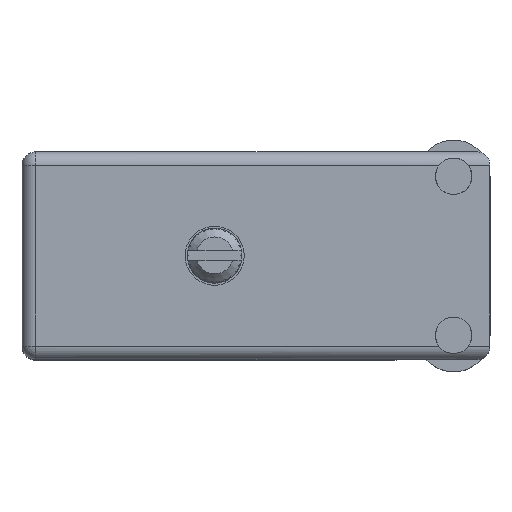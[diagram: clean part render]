
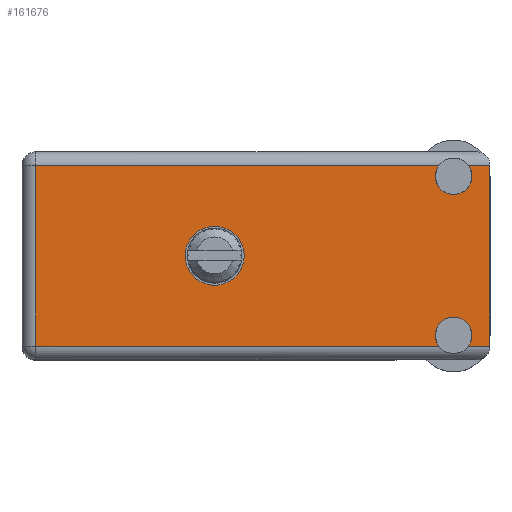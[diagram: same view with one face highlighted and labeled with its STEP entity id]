
A CAD part, top view. The second image highlights one B-rep face of the part: STEP entity #161676.
In plain terms, the highlighted face is planar.
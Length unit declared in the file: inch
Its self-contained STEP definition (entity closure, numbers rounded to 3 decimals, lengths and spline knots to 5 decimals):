
#1662 = DIRECTION ( 'NONE',  ( 1., 0., 0. ) ) ;
#2091 = VECTOR ( 'NONE', #37955, 39.37008 ) ;
#2223 = CIRCLE ( 'NONE', #14769, 0.1015 ) ;
#3680 = DIRECTION ( 'NONE',  ( 0., 0., 1. ) ) ;
#5959 = VERTEX_POINT ( 'NONE', #51425 ) ;
#6111 = FACE_BOUND ( 'NONE', #151323, .T. ) ;
#6611 = CARTESIAN_POINT ( 'NONE',  ( 1.484, 0.906, -0.084 ) ) ;
#6957 = CARTESIAN_POINT ( 'NONE',  ( 1.53437, 0.906, -0.668 ) ) ;
#7095 = DIRECTION ( 'NONE',  ( -1., 0., 0. ) ) ;
#10945 = EDGE_CURVE ( 'NONE', #169000, #53240, #169586, .T. ) ;
#13604 = ORIENTED_EDGE ( 'NONE', *, *, #43337, .T. ) ;
#13676 = CARTESIAN_POINT ( 'NONE',  ( 1.484, 0.906, -0.1465 ) ) ;
#14152 = EDGE_CURVE ( 'NONE', #182163, #169000, #41127, .T. ) ;
#14405 = AXIS2_PLACEMENT_3D ( 'NONE', #101780, #162920, #118537 ) ;
#14769 = AXIS2_PLACEMENT_3D ( 'NONE', #75644, #45050, #132971 ) ;
#16788 = CIRCLE ( 'NONE', #189919, 0.0625 ) ;
#18966 = DIRECTION ( 'NONE',  ( 0., 0., 1. ) ) ;
#21235 = DIRECTION ( 'NONE',  ( 0., 0., 1. ) ) ;
#26805 = AXIS2_PLACEMENT_3D ( 'NONE', #66387, #154219, #18966 ) ;
#27345 = DIRECTION ( 'NONE',  ( 1., 0., 0. ) ) ;
#29380 = CARTESIAN_POINT ( 'NONE',  ( 1.609, 0.906, -0.047 ) ) ;
#34999 = CARTESIAN_POINT ( 'NONE',  ( 0.047, 0.906, -0.715 ) ) ;
#36084 = DIRECTION ( 'NONE',  ( 0., 1., 0. ) ) ;
#37955 = DIRECTION ( 'NONE',  ( 0., 0., 1. ) ) ;
#38974 = CARTESIAN_POINT ( 'NONE',  ( 0.047, 0.906, -0.668 ) ) ;
#39924 = CIRCLE ( 'NONE', #125039, 0.1015 ) ;
#40040 = ORIENTED_EDGE ( 'NONE', *, *, #151845, .F. ) ;
#41127 = CIRCLE ( 'NONE', #79023, 0.0625 ) ;
#43337 = EDGE_CURVE ( 'NONE', #182163, #186503, #110846, .T. ) ;
#44783 = DIRECTION ( 'NONE',  ( 0., 1., 0. ) ) ;
#45050 = DIRECTION ( 'NONE',  ( 0., 1., 0. ) ) ;
#45197 = EDGE_CURVE ( 'NONE', #61431, #184774, #151283, .T. ) ;
#45761 = DIRECTION ( 'NONE',  ( 0., 0., 1. ) ) ;
#49197 = VERTEX_POINT ( 'NONE', #66210 ) ;
#49607 = FACE_OUTER_BOUND ( 'NONE', #87204, .T. ) ;
#50571 = CARTESIAN_POINT ( 'NONE',  ( 0.6625, 0.906, -0.256 ) ) ;
#51425 = CARTESIAN_POINT ( 'NONE',  ( 1.609, 0.906, -0.047 ) ) ;
#51627 = DIRECTION ( 'NONE',  ( 0., 1., 0. ) ) ;
#51760 = LINE ( 'NONE', #34999, #2091 ) ;
#53240 = VERTEX_POINT ( 'NONE', #6957 ) ;
#54819 = DIRECTION ( 'NONE',  ( -1., 0., 0. ) ) ;
#59833 = VECTOR ( 'NONE', #7095, 39.37008 ) ;
#61431 = VERTEX_POINT ( 'NONE', #144562 ) ;
#61825 = VERTEX_POINT ( 'NONE', #50571 ) ;
#61921 = EDGE_CURVE ( 'NONE', #184774, #67930, #16788, .T. ) ;
#63448 = ORIENTED_EDGE ( 'NONE', *, *, #10945, .F. ) ;
#66210 = CARTESIAN_POINT ( 'NONE',  ( 0.047, 0.906, -0.047 ) ) ;
#66387 = CARTESIAN_POINT ( 'NONE',  ( 0., 0.906, -0.715 ) ) ;
#67930 = VERTEX_POINT ( 'NONE', #141835 ) ;
#70359 = CARTESIAN_POINT ( 'NONE',  ( 1.484, 0.906, -0.084 ) ) ;
#73168 = ORIENTED_EDGE ( 'NONE', *, *, #86014, .F. ) ;
#75644 = CARTESIAN_POINT ( 'NONE',  ( 0.6625, 0.906, -0.3575 ) ) ;
#76755 = LINE ( 'NONE', #29380, #187191 ) ;
#79023 = AXIS2_PLACEMENT_3D ( 'NONE', #184131, #36084, #21235 ) ;
#84676 = CARTESIAN_POINT ( 'NONE',  ( 1.609, 0.906, -0.047 ) ) ;
#86014 = EDGE_CURVE ( 'NONE', #150300, #5959, #179741, .T. ) ;
#87204 = EDGE_LOOP ( 'NONE', ( #182590, #155011, #193056, #114177, #73168, #184280, #63448, #105481, #13604, #168948 ) ) ;
#88537 = EDGE_CURVE ( 'NONE', #150300, #53240, #160404, .T. ) ;
#92865 = DIRECTION ( 'NONE',  ( 0., 0., 1. ) ) ;
#95517 = DIRECTION ( 'NONE',  ( 0., 1., 0. ) ) ;
#96974 = PLANE ( 'NONE',  #26805 ) ;
#100883 = AXIS2_PLACEMENT_3D ( 'NONE', #70359, #51627, #111887 ) ;
#101435 = LINE ( 'NONE', #84676, #102736 ) ;
#101780 = CARTESIAN_POINT ( 'NONE',  ( 1.484, 0.906, -0.631 ) ) ;
#102736 = VECTOR ( 'NONE', #27345, 39.37008 ) ;
#105481 = ORIENTED_EDGE ( 'NONE', *, *, #14152, .F. ) ;
#105978 = EDGE_CURVE ( 'NONE', #61431, #5959, #101435, .T. ) ;
#107189 = VECTOR ( 'NONE', #54819, 39.37008 ) ;
#110846 = LINE ( 'NONE', #158134, #59833 ) ;
#111887 = DIRECTION ( 'NONE',  ( 0., 0., 1. ) ) ;
#112144 = CARTESIAN_POINT ( 'NONE',  ( 0., 0.906, -0.668 ) ) ;
#114177 = ORIENTED_EDGE ( 'NONE', *, *, #105978, .T. ) ;
#118537 = DIRECTION ( 'NONE',  ( 0., 0., 1. ) ) ;
#125039 = AXIS2_PLACEMENT_3D ( 'NONE', #166171, #44783, #45761 ) ;
#126392 = EDGE_CURVE ( 'NONE', #49197, #67930, #76755, .T. ) ;
#131061 = ORIENTED_EDGE ( 'NONE', *, *, #175095, .F. ) ;
#132971 = DIRECTION ( 'NONE',  ( 0., 0., 1. ) ) ;
#133294 = CARTESIAN_POINT ( 'NONE',  ( 1.609, 0.906, -0.668 ) ) ;
#141835 = CARTESIAN_POINT ( 'NONE',  ( 1.43363, 0.906, -0.047 ) ) ;
#144562 = CARTESIAN_POINT ( 'NONE',  ( 1.53437, 0.906, -0.047 ) ) ;
#150300 = VERTEX_POINT ( 'NONE', #133294 ) ;
#151283 = CIRCLE ( 'NONE', #100883, 0.0625 ) ;
#151323 = EDGE_LOOP ( 'NONE', ( #131061, #40040 ) ) ;
#151845 = EDGE_CURVE ( 'NONE', #170573, #61825, #2223, .T. ) ;
#154219 = DIRECTION ( 'NONE',  ( 0., 1., 0. ) ) ;
#155011 = ORIENTED_EDGE ( 'NONE', *, *, #61921, .F. ) ;
#158134 = CARTESIAN_POINT ( 'NONE',  ( 0., 0.906, -0.668 ) ) ;
#160404 = LINE ( 'NONE', #112144, #107189 ) ;
#161676 = ADVANCED_FACE ( 'NONE', ( #6111, #49607 ), #96974, .T. ) ;
#162920 = DIRECTION ( 'NONE',  ( 0., 1., 0. ) ) ;
#163798 = VECTOR ( 'NONE', #92865, 39.37008 ) ;
#164957 = CARTESIAN_POINT ( 'NONE',  ( 1.609, 0.906, 0. ) ) ;
#166171 = CARTESIAN_POINT ( 'NONE',  ( 0.6625, 0.906, -0.3575 ) ) ;
#166522 = CARTESIAN_POINT ( 'NONE',  ( 0.6625, 0.906, -0.459 ) ) ;
#168948 = ORIENTED_EDGE ( 'NONE', *, *, #178101, .T. ) ;
#169000 = VERTEX_POINT ( 'NONE', #185958 ) ;
#169586 = CIRCLE ( 'NONE', #14405, 0.0625 ) ;
#170573 = VERTEX_POINT ( 'NONE', #166522 ) ;
#175095 = EDGE_CURVE ( 'NONE', #61825, #170573, #39924, .T. ) ;
#178101 = EDGE_CURVE ( 'NONE', #186503, #49197, #51760, .T. ) ;
#179741 = LINE ( 'NONE', #164957, #163798 ) ;
#182163 = VERTEX_POINT ( 'NONE', #193213 ) ;
#182590 = ORIENTED_EDGE ( 'NONE', *, *, #126392, .T. ) ;
#184131 = CARTESIAN_POINT ( 'NONE',  ( 1.484, 0.906, -0.631 ) ) ;
#184280 = ORIENTED_EDGE ( 'NONE', *, *, #88537, .T. ) ;
#184774 = VERTEX_POINT ( 'NONE', #13676 ) ;
#185958 = CARTESIAN_POINT ( 'NONE',  ( 1.484, 0.906, -0.5685 ) ) ;
#186503 = VERTEX_POINT ( 'NONE', #38974 ) ;
#187191 = VECTOR ( 'NONE', #1662, 39.37008 ) ;
#189919 = AXIS2_PLACEMENT_3D ( 'NONE', #6611, #95517, #3680 ) ;
#193056 = ORIENTED_EDGE ( 'NONE', *, *, #45197, .F. ) ;
#193213 = CARTESIAN_POINT ( 'NONE',  ( 1.43363, 0.906, -0.668 ) ) ;
